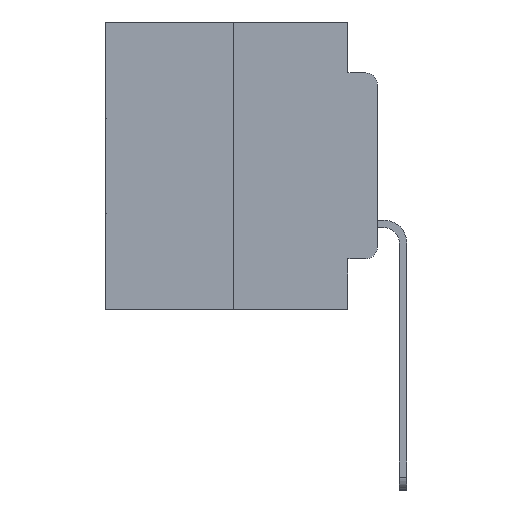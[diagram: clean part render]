
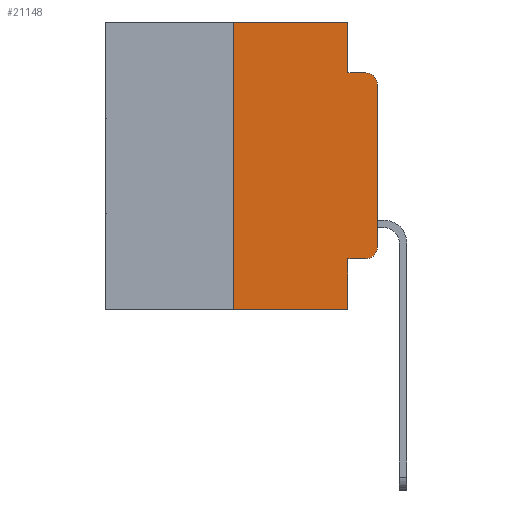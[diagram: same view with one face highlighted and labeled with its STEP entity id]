
A CAD part, left-side view. The second image highlights one B-rep face of the part: STEP entity #21148.
In plain terms, the highlighted planar face has unit normal (-1, 0, 0).
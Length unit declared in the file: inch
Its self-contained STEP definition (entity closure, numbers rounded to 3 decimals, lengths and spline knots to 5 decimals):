
#91 = VERTEX_POINT ( 'NONE', #19687 ) ;
#981 = VECTOR ( 'NONE', #21077, 39.37008 ) ;
#1516 = DIRECTION ( 'NONE',  ( 0., 0., 1. ) ) ;
#1694 = CARTESIAN_POINT ( 'NONE',  ( 0., 0.051, -0.0885 ) ) ;
#1978 = ORIENTED_EDGE ( 'NONE', *, *, #14626, .T. ) ;
#1979 = LINE ( 'NONE', #21368, #12559 ) ;
#2041 = ORIENTED_EDGE ( 'NONE', *, *, #24655, .T. ) ;
#2290 = ORIENTED_EDGE ( 'NONE', *, *, #18316, .F. ) ;
#2856 = DIRECTION ( 'NONE',  ( 0., 0., 1. ) ) ;
#3042 = ORIENTED_EDGE ( 'NONE', *, *, #4804, .T. ) ;
#3168 = VERTEX_POINT ( 'NONE', #22937 ) ;
#3883 = CARTESIAN_POINT ( 'NONE',  ( 0., 0.02, -0.3915 ) ) ;
#4042 = DIRECTION ( 'NONE',  ( 0., -1., 0. ) ) ;
#4070 = DIRECTION ( 'NONE',  ( 1., 0., 0. ) ) ;
#4721 = ORIENTED_EDGE ( 'NONE', *, *, #13480, .F. ) ;
#4804 = EDGE_CURVE ( 'NONE', #15509, #18613, #1979, .T. ) ;
#4825 = ORIENTED_EDGE ( 'NONE', *, *, #25983, .T. ) ;
#4973 = VERTEX_POINT ( 'NONE', #26358 ) ;
#5088 = VECTOR ( 'NONE', #21572, 39.37008 ) ;
#5489 = EDGE_CURVE ( 'NONE', #19907, #91, #17347, .T. ) ;
#5644 = ORIENTED_EDGE ( 'NONE', *, *, #17754, .F. ) ;
#5818 = CARTESIAN_POINT ( 'NONE',  ( 0., 0.051, 0. ) ) ;
#5949 = DIRECTION ( 'NONE',  ( 0., -1., 0. ) ) ;
#6029 = CARTESIAN_POINT ( 'NONE',  ( 0., 0.051, -0.4115 ) ) ;
#6195 = DIRECTION ( 'NONE',  ( 0., 0., -1. ) ) ;
#7250 = AXIS2_PLACEMENT_3D ( 'NONE', #17385, #4070, #19583 ) ;
#7830 = LINE ( 'NONE', #25434, #981 ) ;
#7957 = LINE ( 'NONE', #25817, #24091 ) ;
#9635 = VECTOR ( 'NONE', #16495, 39.37008 ) ;
#9652 = VECTOR ( 'NONE', #4042, 39.37008 ) ;
#11050 = LINE ( 'NONE', #15015, #5088 ) ;
#11382 = EDGE_LOOP ( 'NONE', ( #1978, #2041, #2290, #22692, #18553, #5644, #4825, #4721, #3042, #18604 ) ) ;
#11705 = CIRCLE ( 'NONE', #14649, 0.02 ) ;
#12468 = DIRECTION ( 'NONE',  ( -1., 0., 0. ) ) ;
#12559 = VECTOR ( 'NONE', #5949, 39.37008 ) ;
#12925 = DIRECTION ( 'NONE',  ( 0., 0., -1. ) ) ;
#12963 = VERTEX_POINT ( 'NONE', #14536 ) ;
#13105 = CARTESIAN_POINT ( 'NONE',  ( 0., 0.25, 0. ) ) ;
#13304 = VERTEX_POINT ( 'NONE', #22611 ) ;
#13480 = EDGE_CURVE ( 'NONE', #15509, #12963, #7830, .T. ) ;
#13648 = VERTEX_POINT ( 'NONE', #21640 ) ;
#14305 = CARTESIAN_POINT ( 'NONE',  ( 0., 0.473, 0. ) ) ;
#14536 = CARTESIAN_POINT ( 'NONE',  ( 0., 0.051, -0.5 ) ) ;
#14626 = EDGE_CURVE ( 'NONE', #13304, #4973, #22573, .T. ) ;
#14649 = AXIS2_PLACEMENT_3D ( 'NONE', #3883, #19426, #6195 ) ;
#15015 = CARTESIAN_POINT ( 'NONE',  ( 0., 0.473, -0.5 ) ) ;
#15509 = VERTEX_POINT ( 'NONE', #6029 ) ;
#15682 = CIRCLE ( 'NONE', #21319, 0.02 ) ;
#16213 = LINE ( 'NONE', #1694, #9652 ) ;
#16344 = CARTESIAN_POINT ( 'NONE',  ( 0., 0., 0. ) ) ;
#16495 = DIRECTION ( 'NONE',  ( 0., -1., 0. ) ) ;
#17347 = LINE ( 'NONE', #27957, #28089 ) ;
#17385 = CARTESIAN_POINT ( 'NONE',  ( 0., 0.473, 0. ) ) ;
#17754 = EDGE_CURVE ( 'NONE', #3168, #20639, #7957, .T. ) ;
#18316 = EDGE_CURVE ( 'NONE', #91, #13648, #16213, .T. ) ;
#18553 = ORIENTED_EDGE ( 'NONE', *, *, #26424, .F. ) ;
#18604 = ORIENTED_EDGE ( 'NONE', *, *, #18676, .T. ) ;
#18613 = VERTEX_POINT ( 'NONE', #23438 ) ;
#18676 = EDGE_CURVE ( 'NONE', #18613, #13304, #11705, .T. ) ;
#19426 = DIRECTION ( 'NONE',  ( -1., 0., 0. ) ) ;
#19583 = DIRECTION ( 'NONE',  ( 0., 0., -1. ) ) ;
#19687 = CARTESIAN_POINT ( 'NONE',  ( 0., 0.051, -0.0885 ) ) ;
#19907 = VERTEX_POINT ( 'NONE', #5818 ) ;
#20639 = VERTEX_POINT ( 'NONE', #13105 ) ;
#21077 = DIRECTION ( 'NONE',  ( 0., 0., -1. ) ) ;
#21148 = ADVANCED_FACE ( 'NONE', ( #28311 ), #28085, .F. ) ;
#21319 = AXIS2_PLACEMENT_3D ( 'NONE', #25524, #12468, #27625 ) ;
#21368 = CARTESIAN_POINT ( 'NONE',  ( 0., 0.051, -0.4115 ) ) ;
#21572 = DIRECTION ( 'NONE',  ( 0., -1., 0. ) ) ;
#21640 = CARTESIAN_POINT ( 'NONE',  ( 0., 0.02, -0.0885 ) ) ;
#22573 = LINE ( 'NONE', #16344, #28218 ) ;
#22611 = CARTESIAN_POINT ( 'NONE',  ( 0., 0., -0.3915 ) ) ;
#22692 = ORIENTED_EDGE ( 'NONE', *, *, #5489, .F. ) ;
#22937 = CARTESIAN_POINT ( 'NONE',  ( 0., 0.25, -0.5 ) ) ;
#23438 = CARTESIAN_POINT ( 'NONE',  ( 0., 0.02, -0.4115 ) ) ;
#24091 = VECTOR ( 'NONE', #1516, 39.37008 ) ;
#24655 = EDGE_CURVE ( 'NONE', #4973, #13648, #15682, .T. ) ;
#25434 = CARTESIAN_POINT ( 'NONE',  ( 0., 0.051, 0. ) ) ;
#25524 = CARTESIAN_POINT ( 'NONE',  ( 0., 0.02, -0.1085 ) ) ;
#25817 = CARTESIAN_POINT ( 'NONE',  ( 0., 0.25, 0. ) ) ;
#25983 = EDGE_CURVE ( 'NONE', #3168, #12963, #11050, .T. ) ;
#26358 = CARTESIAN_POINT ( 'NONE',  ( 0., 0., -0.1085 ) ) ;
#26424 = EDGE_CURVE ( 'NONE', #20639, #19907, #27016, .T. ) ;
#27016 = LINE ( 'NONE', #14305, #9635 ) ;
#27625 = DIRECTION ( 'NONE',  ( 0., 0., -1. ) ) ;
#27957 = CARTESIAN_POINT ( 'NONE',  ( 0., 0.051, 0. ) ) ;
#28085 = PLANE ( 'NONE',  #7250 ) ;
#28089 = VECTOR ( 'NONE', #12925, 39.37008 ) ;
#28218 = VECTOR ( 'NONE', #2856, 39.37008 ) ;
#28311 = FACE_OUTER_BOUND ( 'NONE', #11382, .T. ) ;
